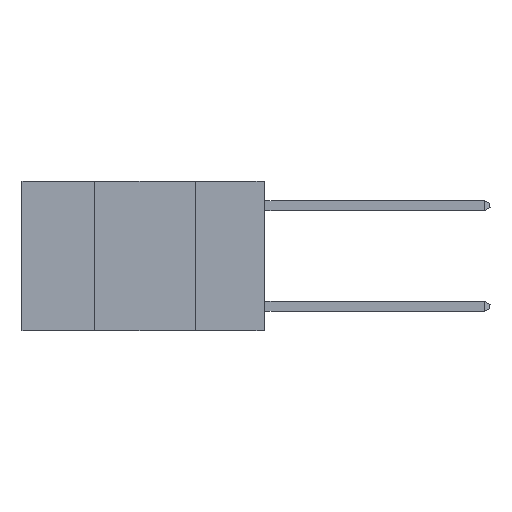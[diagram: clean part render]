
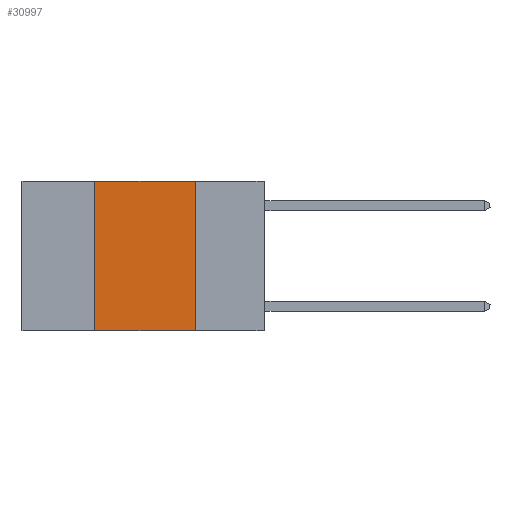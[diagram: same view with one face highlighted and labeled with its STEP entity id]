
A CAD part, left-side view. The second image highlights one B-rep face of the part: STEP entity #30997.
In plain terms, the highlighted planar face has unit normal (-1, 0, 0).
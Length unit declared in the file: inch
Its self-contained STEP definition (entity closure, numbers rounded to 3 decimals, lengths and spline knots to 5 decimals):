
#738 = CARTESIAN_POINT ( 'NONE',  ( 0., 0.6, -0.37 ) ) ;
#1703 = VERTEX_POINT ( 'NONE', #14984 ) ;
#2471 = ORIENTED_EDGE ( 'NONE', *, *, #18566, .F. ) ;
#3270 = DIRECTION ( 'NONE',  ( 0., -1., 0. ) ) ;
#3880 = VECTOR ( 'NONE', #26640, 39.37008 ) ;
#4455 = VERTEX_POINT ( 'NONE', #23368 ) ;
#4466 = DIRECTION ( 'NONE',  ( 1., 0., 0. ) ) ;
#8368 = VECTOR ( 'NONE', #28587, 39.37008 ) ;
#8423 = LINE ( 'NONE', #23190, #20677 ) ;
#9256 = CARTESIAN_POINT ( 'NONE',  ( 0., 0.17, 0. ) ) ;
#10065 = LINE ( 'NONE', #738, #22272 ) ;
#13424 = ORIENTED_EDGE ( 'NONE', *, *, #19419, .F. ) ;
#14781 = VERTEX_POINT ( 'NONE', #9256 ) ;
#14984 = CARTESIAN_POINT ( 'NONE',  ( 0., 0.42, 0. ) ) ;
#15710 = ORIENTED_EDGE ( 'NONE', *, *, #29076, .F. ) ;
#17080 = LINE ( 'NONE', #24232, #3880 ) ;
#17462 = CARTESIAN_POINT ( 'NONE',  ( 0., 0.17, -0.37 ) ) ;
#18566 = EDGE_CURVE ( 'NONE', #1703, #14781, #8423, .T. ) ;
#19000 = VERTEX_POINT ( 'NONE', #17462 ) ;
#19264 = CARTESIAN_POINT ( 'NONE',  ( 0., 0.6, 0. ) ) ;
#19419 = EDGE_CURVE ( 'NONE', #14781, #19000, #30017, .T. ) ;
#20677 = VECTOR ( 'NONE', #25645, 39.37008 ) ;
#21691 = DIRECTION ( 'NONE',  ( 0., 0., -1. ) ) ;
#22272 = VECTOR ( 'NONE', #3270, 39.37008 ) ;
#23190 = CARTESIAN_POINT ( 'NONE',  ( 0., 0.6, 0. ) ) ;
#23368 = CARTESIAN_POINT ( 'NONE',  ( 0., 0.42, -0.37 ) ) ;
#24232 = CARTESIAN_POINT ( 'NONE',  ( 0., 0.42, 0. ) ) ;
#25645 = DIRECTION ( 'NONE',  ( 0., -1., 0. ) ) ;
#26015 = FACE_OUTER_BOUND ( 'NONE', #27449, .T. ) ;
#26224 = CARTESIAN_POINT ( 'NONE',  ( 0., 0.17, 0. ) ) ;
#26640 = DIRECTION ( 'NONE',  ( 0., 0., 1. ) ) ;
#27449 = EDGE_LOOP ( 'NONE', ( #13424, #2471, #15710, #29275 ) ) ;
#28587 = DIRECTION ( 'NONE',  ( 0., 0., -1. ) ) ;
#28816 = PLANE ( 'NONE',  #30528 ) ;
#29076 = EDGE_CURVE ( 'NONE', #4455, #1703, #17080, .T. ) ;
#29275 = ORIENTED_EDGE ( 'NONE', *, *, #30670, .T. ) ;
#30017 = LINE ( 'NONE', #26224, #8368 ) ;
#30528 = AXIS2_PLACEMENT_3D ( 'NONE', #19264, #4466, #21691 ) ;
#30670 = EDGE_CURVE ( 'NONE', #4455, #19000, #10065, .T. ) ;
#30997 = ADVANCED_FACE ( 'NONE', ( #26015 ), #28816, .F. ) ;
